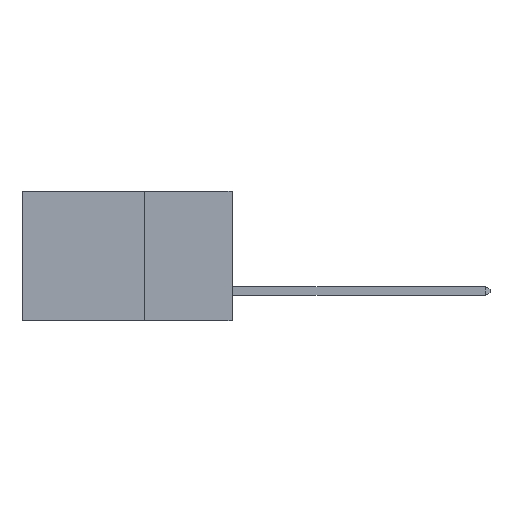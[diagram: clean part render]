
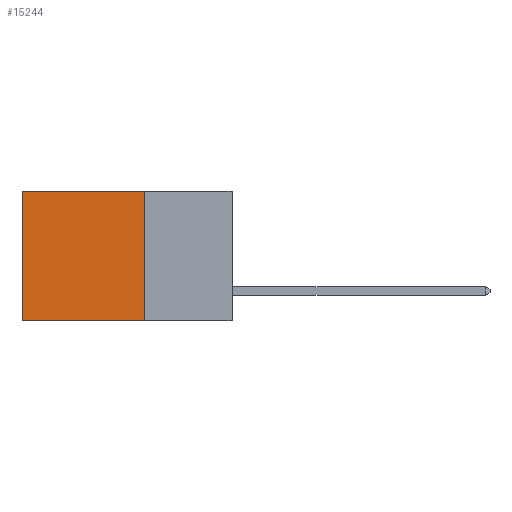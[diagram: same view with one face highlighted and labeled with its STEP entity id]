
A CAD part, left-side view. The second image highlights one B-rep face of the part: STEP entity #15244.
In plain terms, the highlighted planar face has unit normal (-1, 0, 0).
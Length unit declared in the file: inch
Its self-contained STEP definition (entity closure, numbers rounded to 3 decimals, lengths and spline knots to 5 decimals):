
#340 = CARTESIAN_POINT ( 'NONE',  ( 0.2875, 0.6, 0. ) ) ;
#344 = CARTESIAN_POINT ( 'NONE',  ( 0.2875, 0.25, 0. ) ) ;
#2181 = DIRECTION ( 'NONE',  ( 0., 0., -1. ) ) ;
#2240 = CARTESIAN_POINT ( 'NONE',  ( 0.2875, 0.25, 0. ) ) ;
#3466 = VECTOR ( 'NONE', #4937, 39.37008 ) ;
#4045 = DIRECTION ( 'NONE',  ( 0., 1., 0. ) ) ;
#4937 = DIRECTION ( 'NONE',  ( 0., 1., 0. ) ) ;
#5101 = LINE ( 'NONE', #16156, #13748 ) ;
#5995 = LINE ( 'NONE', #2240, #14597 ) ;
#8766 = AXIS2_PLACEMENT_3D ( 'NONE', #344, #12683, #2181 ) ;
#8897 = EDGE_CURVE ( 'NONE', #13274, #18048, #5995, .T. ) ;
#9182 = VERTEX_POINT ( 'NONE', #13451 ) ;
#9276 = PLANE ( 'NONE',  #8766 ) ;
#9575 = EDGE_CURVE ( 'NONE', #18048, #21160, #5101, .T. ) ;
#9607 = ORIENTED_EDGE ( 'NONE', *, *, #8897, .T. ) ;
#9898 = ORIENTED_EDGE ( 'NONE', *, *, #12536, .F. ) ;
#12401 = ORIENTED_EDGE ( 'NONE', *, *, #9575, .T. ) ;
#12536 = EDGE_CURVE ( 'NONE', #9182, #21160, #12769, .T. ) ;
#12683 = DIRECTION ( 'NONE',  ( 1., 0., 0. ) ) ;
#12769 = LINE ( 'NONE', #21898, #3466 ) ;
#13274 = VERTEX_POINT ( 'NONE', #20550 ) ;
#13451 = CARTESIAN_POINT ( 'NONE',  ( 0.2875, 0.25, -0.37 ) ) ;
#13748 = VECTOR ( 'NONE', #17827, 39.37008 ) ;
#14164 = EDGE_LOOP ( 'NONE', ( #12401, #9898, #15775, #9607 ) ) ;
#14597 = VECTOR ( 'NONE', #4045, 39.37008 ) ;
#15039 = FACE_OUTER_BOUND ( 'NONE', #14164, .T. ) ;
#15244 = ADVANCED_FACE ( 'NONE', ( #15039 ), #9276, .F. ) ;
#15775 = ORIENTED_EDGE ( 'NONE', *, *, #18307, .F. ) ;
#16156 = CARTESIAN_POINT ( 'NONE',  ( 0.2875, 0.6, 0. ) ) ;
#16713 = CARTESIAN_POINT ( 'NONE',  ( 0.2875, 0.25, 0. ) ) ;
#17827 = DIRECTION ( 'NONE',  ( 0., 0., -1. ) ) ;
#18048 = VERTEX_POINT ( 'NONE', #340 ) ;
#18307 = EDGE_CURVE ( 'NONE', #13274, #9182, #18581, .T. ) ;
#18581 = LINE ( 'NONE', #16713, #21971 ) ;
#20550 = CARTESIAN_POINT ( 'NONE',  ( 0.2875, 0.25, 0. ) ) ;
#21160 = VERTEX_POINT ( 'NONE', #22294 ) ;
#21733 = DIRECTION ( 'NONE',  ( 0., 0., -1. ) ) ;
#21898 = CARTESIAN_POINT ( 'NONE',  ( 0.2875, 0.25, -0.37 ) ) ;
#21971 = VECTOR ( 'NONE', #21733, 39.37008 ) ;
#22294 = CARTESIAN_POINT ( 'NONE',  ( 0.2875, 0.6, -0.37 ) ) ;
